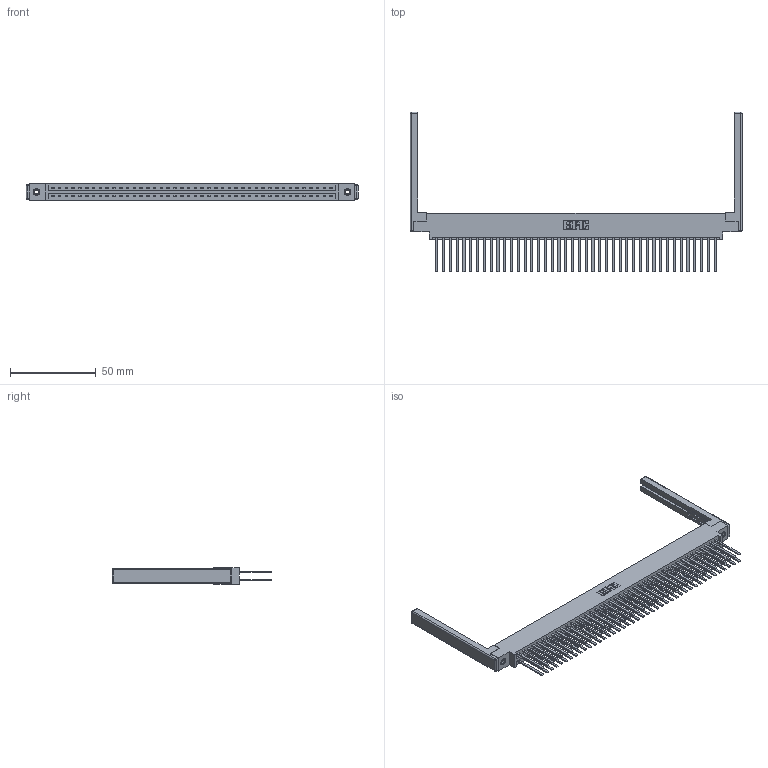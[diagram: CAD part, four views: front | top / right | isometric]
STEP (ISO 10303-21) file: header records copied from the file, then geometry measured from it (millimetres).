
FILE_DESCRIPTION (( 'STEP AP203' ), '1' );
FILE_NAME ('387-084-544-868.STEP', '2019-10-23T01:53:39', ( '' ), ( '' ), 'SwSTEP 2.0', 'SolidWorks 2016', '' );
FILE_SCHEMA (( 'CONFIG_CONTROL_DESIGN' ));
Length unit declared in the file: inch
Products named in the file (5): 307-220-068; 337 Part_0.170 Offset - 0.156 Dia-TI; 345-292-001_345-293-144; 345-250-001_345-250-001-102; 387-084-544-868
Assembly tree (89 placements, depth 2):
  387-084-544-868
    337 Part_0.170 Offset - 0.156 Dia-TI
    345-292-001_345-293-144  x84
    345-250-001_345-250-001-102  x2
    307-220-068  x2
Bounding box: 193.85 x 93.35 x 9.4 mm (x, y, z)
Volume: 25874.6 mm3; surface area: 32283.1 mm2
Topology: 89 solids, 89 shells, 4304 faces, 12725 edges, 8350 vertices
Faces by surface type: plane 3018, cylinder 1262, cone 12, sphere 8, torus 4
Entity records: 35272 total; most frequent: CARTESIAN_POINT 5907, ORIENTED_EDGE 5832, DIRECTION 5090, EDGE_CURVE 2916, LINE 2742, VECTOR 2742, VERTEX_POINT 1934, AXIS2_PLACEMENT_3D 1174
